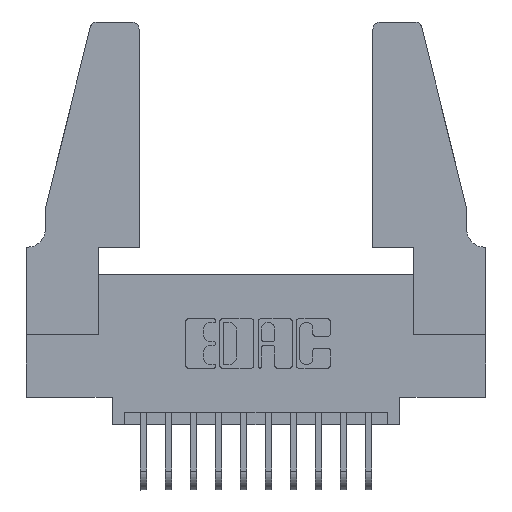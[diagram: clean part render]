
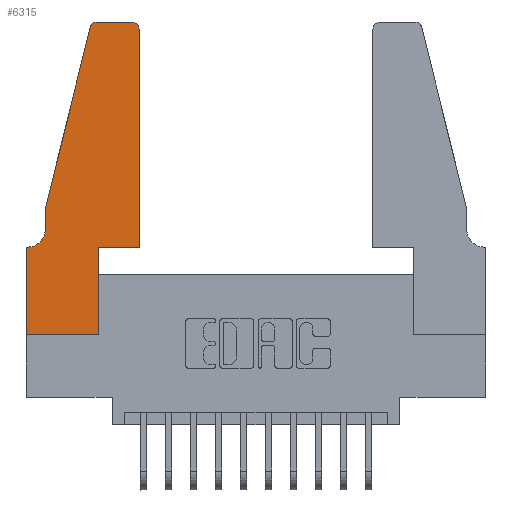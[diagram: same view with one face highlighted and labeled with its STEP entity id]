
A CAD part, top view. The second image highlights one B-rep face of the part: STEP entity #6315.
In plain terms, the highlighted planar face has unit normal (0, 0, 1).
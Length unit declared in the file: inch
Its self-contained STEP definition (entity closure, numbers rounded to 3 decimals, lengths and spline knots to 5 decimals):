
#99 = AXIS2_PLACEMENT_3D ( 'NONE', #12696, #10438, #1381 ) ;
#118 = CARTESIAN_POINT ( 'NONE',  ( 0.2865, 0.35, 0.37 ) ) ;
#130 = AXIS2_PLACEMENT_3D ( 'NONE', #3077, #10775, #4190 ) ;
#274 = EDGE_CURVE ( 'NONE', #6218, #8075, #12029, .T. ) ;
#400 = PLANE ( 'NONE',  #8371 ) ;
#440 = EDGE_CURVE ( 'NONE', #8025, #13500, #1206, .T. ) ;
#605 = CARTESIAN_POINT ( 'NONE',  ( 0.0755, 0.35, 0.37 ) ) ;
#658 = EDGE_LOOP ( 'NONE', ( #12128, #10981, #8929, #5956, #7923, #12804, #10598, #2861, #9734, #8048, #9605, #10264 ) ) ;
#904 = CARTESIAN_POINT ( 'NONE',  ( 0.0755, 0.42, 0.37 ) ) ;
#908 = CARTESIAN_POINT ( 'NONE',  ( 0.0755, 0.5, 0.37 ) ) ;
#928 = EDGE_CURVE ( 'NONE', #5906, #6136, #3265, .T. ) ;
#1037 = CIRCLE ( 'NONE', #130, 0.07 ) ;
#1045 = CIRCLE ( 'NONE', #7193, 0.03 ) ;
#1095 = VECTOR ( 'NONE', #3205, 39.37008 ) ;
#1198 = CARTESIAN_POINT ( 'NONE',  ( 0.4205, 1.22, 0.37 ) ) ;
#1206 = CIRCLE ( 'NONE', #99, 0.03 ) ;
#1381 = DIRECTION ( 'NONE',  ( 1., 0., 0. ) ) ;
#1518 = DIRECTION ( 'NONE',  ( 0., 0., 1. ) ) ;
#1726 = VECTOR ( 'NONE', #7624, 39.37008 ) ;
#2010 = DIRECTION ( 'NONE',  ( -0.239, -0.971, 0. ) ) ;
#2196 = LINE ( 'NONE', #5158, #13176 ) ;
#2294 = DIRECTION ( 'NONE',  ( 1., 0., 0. ) ) ;
#2644 = CARTESIAN_POINT ( 'NONE',  ( 0.4505, 0.35, 0.37 ) ) ;
#2861 = ORIENTED_EDGE ( 'NONE', *, *, #14203, .T. ) ;
#3067 = CARTESIAN_POINT ( 'NONE',  ( 0.284, 1.25, 0.37 ) ) ;
#3077 = CARTESIAN_POINT ( 'NONE',  ( 0.0055, 0.42, 0.37 ) ) ;
#3205 = DIRECTION ( 'NONE',  ( 0., 1., 0. ) ) ;
#3217 = CARTESIAN_POINT ( 'NONE',  ( 0., 0., 0.37 ) ) ;
#3253 = CARTESIAN_POINT ( 'NONE',  ( 0., 0.35, 0.37 ) ) ;
#3265 = LINE ( 'NONE', #11897, #1095 ) ;
#3355 = DIRECTION ( 'NONE',  ( 1., 0., 0. ) ) ;
#3453 = LINE ( 'NONE', #908, #11876 ) ;
#3463 = VERTEX_POINT ( 'NONE', #11857 ) ;
#3762 = DIRECTION ( 'NONE',  ( -1., 0., 0. ) ) ;
#3877 = DIRECTION ( 'NONE',  ( -1., 0., 0. ) ) ;
#4190 = DIRECTION ( 'NONE',  ( -1., 0., 0. ) ) ;
#4212 = VERTEX_POINT ( 'NONE', #6822 ) ;
#4581 = EDGE_CURVE ( 'NONE', #8075, #13240, #1037, .T. ) ;
#4872 = CARTESIAN_POINT ( 'NONE',  ( 0.2605, 1.25, 0.37 ) ) ;
#5158 = CARTESIAN_POINT ( 'NONE',  ( 0., 0., 0.37 ) ) ;
#5240 = CARTESIAN_POINT ( 'NONE',  ( 0.2865, 0., 0.37 ) ) ;
#5281 = CARTESIAN_POINT ( 'NONE',  ( 0.0755, 0.5, 0.37 ) ) ;
#5906 = VERTEX_POINT ( 'NONE', #5240 ) ;
#5956 = ORIENTED_EDGE ( 'NONE', *, *, #274, .T. ) ;
#6136 = VERTEX_POINT ( 'NONE', #118 ) ;
#6218 = VERTEX_POINT ( 'NONE', #9073 ) ;
#6266 = DIRECTION ( 'NONE',  ( 1., 0., 0. ) ) ;
#6315 = ADVANCED_FACE ( 'NONE', ( #13777 ), #400, .T. ) ;
#6565 = VECTOR ( 'NONE', #3355, 39.37008 ) ;
#6822 = CARTESIAN_POINT ( 'NONE',  ( 0.4505, 0.35, 0.37 ) ) ;
#7026 = VERTEX_POINT ( 'NONE', #3253 ) ;
#7193 = AXIS2_PLACEMENT_3D ( 'NONE', #1198, #8903, #2294 ) ;
#7280 = VECTOR ( 'NONE', #10343, 39.37008 ) ;
#7624 = DIRECTION ( 'NONE',  ( 0., -1., 0. ) ) ;
#7675 = CARTESIAN_POINT ( 'NONE',  ( 0.4205, 1.25, 0.37 ) ) ;
#7923 = ORIENTED_EDGE ( 'NONE', *, *, #4581, .T. ) ;
#8025 = VERTEX_POINT ( 'NONE', #3067 ) ;
#8048 = ORIENTED_EDGE ( 'NONE', *, *, #11477, .T. ) ;
#8075 = VERTEX_POINT ( 'NONE', #904 ) ;
#8129 = CARTESIAN_POINT ( 'NONE',  ( 0., 0.35, 0.37 ) ) ;
#8371 = AXIS2_PLACEMENT_3D ( 'NONE', #8129, #1518, #9209 ) ;
#8459 = VERTEX_POINT ( 'NONE', #11756 ) ;
#8903 = DIRECTION ( 'NONE',  ( 0., 0., 1. ) ) ;
#8929 = ORIENTED_EDGE ( 'NONE', *, *, #11314, .T. ) ;
#9013 = VECTOR ( 'NONE', #3762, 39.37008 ) ;
#9073 = CARTESIAN_POINT ( 'NONE',  ( 0.0755, 0.5, 0.37 ) ) ;
#9209 = DIRECTION ( 'NONE',  ( 1., 0., 0. ) ) ;
#9356 = LINE ( 'NONE', #4872, #9013 ) ;
#9605 = ORIENTED_EDGE ( 'NONE', *, *, #11012, .T. ) ;
#9734 = ORIENTED_EDGE ( 'NONE', *, *, #928, .T. ) ;
#9839 = LINE ( 'NONE', #2644, #7280 ) ;
#10055 = EDGE_CURVE ( 'NONE', #12873, #8025, #9356, .T. ) ;
#10264 = ORIENTED_EDGE ( 'NONE', *, *, #11479, .T. ) ;
#10343 = DIRECTION ( 'NONE',  ( 0., 1., 0. ) ) ;
#10438 = DIRECTION ( 'NONE',  ( 0., 0., 1. ) ) ;
#10598 = ORIENTED_EDGE ( 'NONE', *, *, #11388, .T. ) ;
#10775 = DIRECTION ( 'NONE',  ( 0., 0., -1. ) ) ;
#10845 = LINE ( 'NONE', #3217, #1726 ) ;
#10981 = ORIENTED_EDGE ( 'NONE', *, *, #440, .T. ) ;
#11012 = EDGE_CURVE ( 'NONE', #4212, #3463, #9839, .T. ) ;
#11048 = CARTESIAN_POINT ( 'NONE',  ( 0.4505, 0.35, 0.37 ) ) ;
#11224 = CARTESIAN_POINT ( 'NONE',  ( 0.25487, 1.22718, 0.37 ) ) ;
#11314 = EDGE_CURVE ( 'NONE', #13500, #6218, #3453, .T. ) ;
#11388 = EDGE_CURVE ( 'NONE', #7026, #8459, #10845, .T. ) ;
#11477 = EDGE_CURVE ( 'NONE', #6136, #4212, #12375, .T. ) ;
#11479 = EDGE_CURVE ( 'NONE', #3463, #12873, #1045, .T. ) ;
#11525 = LINE ( 'NONE', #605, #13721 ) ;
#11701 = VECTOR ( 'NONE', #13427, 39.37008 ) ;
#11756 = CARTESIAN_POINT ( 'NONE',  ( 0., 0., 0.37 ) ) ;
#11787 = EDGE_CURVE ( 'NONE', #13240, #7026, #11525, .T. ) ;
#11857 = CARTESIAN_POINT ( 'NONE',  ( 0.4505, 1.22, 0.37 ) ) ;
#11876 = VECTOR ( 'NONE', #2010, 39.37008 ) ;
#11897 = CARTESIAN_POINT ( 'NONE',  ( 0.2865, 0.35, 0.37 ) ) ;
#12029 = LINE ( 'NONE', #5281, #11701 ) ;
#12128 = ORIENTED_EDGE ( 'NONE', *, *, #10055, .T. ) ;
#12375 = LINE ( 'NONE', #11048, #6565 ) ;
#12696 = CARTESIAN_POINT ( 'NONE',  ( 0.284, 1.22, 0.37 ) ) ;
#12804 = ORIENTED_EDGE ( 'NONE', *, *, #11787, .T. ) ;
#12873 = VERTEX_POINT ( 'NONE', #7675 ) ;
#12996 = CARTESIAN_POINT ( 'NONE',  ( 0.0055, 0.35, 0.37 ) ) ;
#13176 = VECTOR ( 'NONE', #6266, 39.37008 ) ;
#13240 = VERTEX_POINT ( 'NONE', #12996 ) ;
#13427 = DIRECTION ( 'NONE',  ( 0., -1., 0. ) ) ;
#13500 = VERTEX_POINT ( 'NONE', #11224 ) ;
#13721 = VECTOR ( 'NONE', #3877, 39.37008 ) ;
#13777 = FACE_OUTER_BOUND ( 'NONE', #658, .T. ) ;
#14203 = EDGE_CURVE ( 'NONE', #8459, #5906, #2196, .T. ) ;
